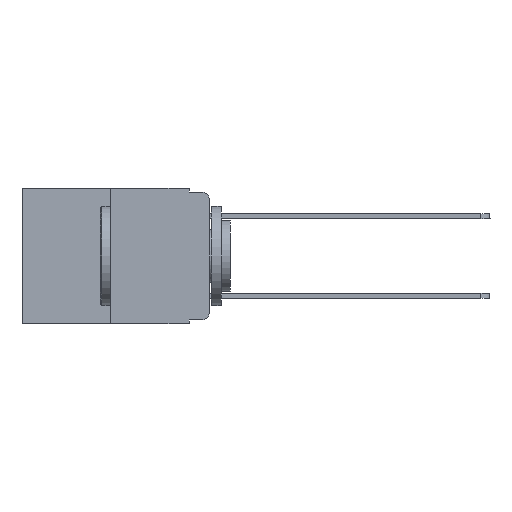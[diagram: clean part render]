
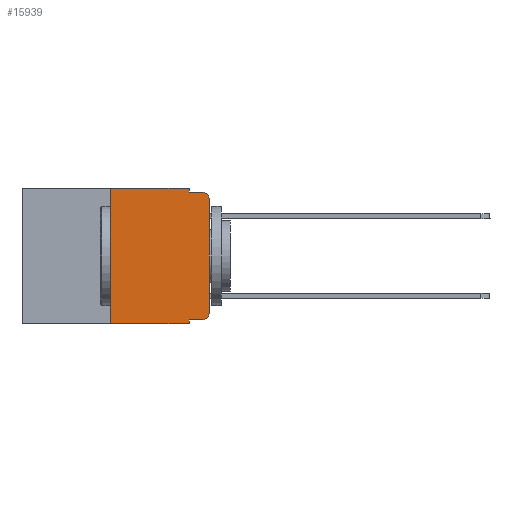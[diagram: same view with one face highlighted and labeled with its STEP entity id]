
A CAD part, left-side view. The second image highlights one B-rep face of the part: STEP entity #15939.
In plain terms, the highlighted planar face has unit normal (-1, 0, 0).
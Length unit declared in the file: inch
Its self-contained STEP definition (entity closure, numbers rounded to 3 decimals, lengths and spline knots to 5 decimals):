
#294 = CARTESIAN_POINT ( 'NONE',  ( 0., 0.02, -0.03 ) ) ;
#412 = CARTESIAN_POINT ( 'NONE',  ( 0., 0.25, 0. ) ) ;
#647 = LINE ( 'NONE', #10317, #19879 ) ;
#972 = VECTOR ( 'NONE', #15878, 39.37008 ) ;
#1545 = EDGE_CURVE ( 'NONE', #7314, #17038, #19181, .T. ) ;
#1686 = VERTEX_POINT ( 'NONE', #6686 ) ;
#2175 = VECTOR ( 'NONE', #7038, 39.37008 ) ;
#2213 = VERTEX_POINT ( 'NONE', #7224 ) ;
#2921 = VECTOR ( 'NONE', #7939, 39.37008 ) ;
#3126 = CIRCLE ( 'NONE', #11602, 0.02 ) ;
#3187 = DIRECTION ( 'NONE',  ( -1., 0., 0. ) ) ;
#3329 = ORIENTED_EDGE ( 'NONE', *, *, #15059, .F. ) ;
#3404 = EDGE_CURVE ( 'NONE', #5990, #1686, #5794, .T. ) ;
#3610 = AXIS2_PLACEMENT_3D ( 'NONE', #5302, #3187, #21129 ) ;
#3692 = CARTESIAN_POINT ( 'NONE',  ( 0., 0.473, -0.343 ) ) ;
#4550 = VECTOR ( 'NONE', #22333, 39.37008 ) ;
#4834 = VERTEX_POINT ( 'NONE', #8156 ) ;
#5104 = VERTEX_POINT ( 'NONE', #17896 ) ;
#5302 = CARTESIAN_POINT ( 'NONE',  ( 0., 0.02, -0.313 ) ) ;
#5708 = ORIENTED_EDGE ( 'NONE', *, *, #1545, .T. ) ;
#5758 = PLANE ( 'NONE',  #7805 ) ;
#5794 = CIRCLE ( 'NONE', #3610, 0.02 ) ;
#5969 = FACE_OUTER_BOUND ( 'NONE', #13307, .T. ) ;
#5990 = VERTEX_POINT ( 'NONE', #6521 ) ;
#6176 = CARTESIAN_POINT ( 'NONE',  ( 0., 0.473, 0. ) ) ;
#6521 = CARTESIAN_POINT ( 'NONE',  ( 0., 0.02, -0.333 ) ) ;
#6523 = CARTESIAN_POINT ( 'NONE',  ( 0., 0.25, -0.343 ) ) ;
#6686 = CARTESIAN_POINT ( 'NONE',  ( 0., 0., -0.313 ) ) ;
#6783 = LINE ( 'NONE', #22415, #4550 ) ;
#6958 = CARTESIAN_POINT ( 'NONE',  ( 0., 0.051, -0.01 ) ) ;
#7038 = DIRECTION ( 'NONE',  ( 0., -1., 0. ) ) ;
#7224 = CARTESIAN_POINT ( 'NONE',  ( 0., 0.051, -0.01 ) ) ;
#7314 = VERTEX_POINT ( 'NONE', #6523 ) ;
#7329 = EDGE_CURVE ( 'NONE', #4834, #5104, #3126, .T. ) ;
#7805 = AXIS2_PLACEMENT_3D ( 'NONE', #9295, #11041, #21880 ) ;
#7939 = DIRECTION ( 'NONE',  ( 0., 0., 1. ) ) ;
#8156 = CARTESIAN_POINT ( 'NONE',  ( 0., 0., -0.03 ) ) ;
#8345 = ORIENTED_EDGE ( 'NONE', *, *, #11212, .F. ) ;
#8813 = LINE ( 'NONE', #9014, #972 ) ;
#9014 = CARTESIAN_POINT ( 'NONE',  ( 0., 0.051, 0. ) ) ;
#9295 = CARTESIAN_POINT ( 'NONE',  ( 0., 0.473, 0. ) ) ;
#9380 = ORIENTED_EDGE ( 'NONE', *, *, #15444, .F. ) ;
#9589 = CARTESIAN_POINT ( 'NONE',  ( 0., 0.051, -0.333 ) ) ;
#10317 = CARTESIAN_POINT ( 'NONE',  ( 0., 0.051, 0. ) ) ;
#11041 = DIRECTION ( 'NONE',  ( 1., 0., 0. ) ) ;
#11212 = EDGE_CURVE ( 'NONE', #15350, #21975, #15100, .T. ) ;
#11302 = ORIENTED_EDGE ( 'NONE', *, *, #12748, .T. ) ;
#11352 = ORIENTED_EDGE ( 'NONE', *, *, #16706, .T. ) ;
#11602 = AXIS2_PLACEMENT_3D ( 'NONE', #294, #21483, #14356 ) ;
#12748 = EDGE_CURVE ( 'NONE', #1686, #4834, #22528, .T. ) ;
#13174 = ORIENTED_EDGE ( 'NONE', *, *, #3404, .T. ) ;
#13307 = EDGE_LOOP ( 'NONE', ( #11302, #13879, #17940, #15015, #8345, #9380, #5708, #3329, #11352, #13174 ) ) ;
#13341 = VECTOR ( 'NONE', #14730, 39.37008 ) ;
#13879 = ORIENTED_EDGE ( 'NONE', *, *, #7329, .T. ) ;
#14356 = DIRECTION ( 'NONE',  ( 0., 0., -1. ) ) ;
#14694 = CARTESIAN_POINT ( 'NONE',  ( 0., 0.25, 0. ) ) ;
#14730 = DIRECTION ( 'NONE',  ( 0., 0., 1. ) ) ;
#15015 = ORIENTED_EDGE ( 'NONE', *, *, #17666, .F. ) ;
#15059 = EDGE_CURVE ( 'NONE', #18977, #17038, #647, .T. ) ;
#15100 = LINE ( 'NONE', #6176, #15673 ) ;
#15132 = EDGE_CURVE ( 'NONE', #2213, #5104, #20431, .T. ) ;
#15350 = VERTEX_POINT ( 'NONE', #14694 ) ;
#15444 = EDGE_CURVE ( 'NONE', #7314, #15350, #16254, .T. ) ;
#15673 = VECTOR ( 'NONE', #20516, 39.37008 ) ;
#15739 = DIRECTION ( 'NONE',  ( 0., 0., -1. ) ) ;
#15809 = CARTESIAN_POINT ( 'NONE',  ( 0., 0.051, 0. ) ) ;
#15878 = DIRECTION ( 'NONE',  ( 0., 0., -1. ) ) ;
#15939 = ADVANCED_FACE ( 'NONE', ( #5969 ), #5758, .F. ) ;
#16025 = VECTOR ( 'NONE', #21160, 39.37008 ) ;
#16254 = LINE ( 'NONE', #412, #2921 ) ;
#16706 = EDGE_CURVE ( 'NONE', #18977, #5990, #6783, .T. ) ;
#17038 = VERTEX_POINT ( 'NONE', #19596 ) ;
#17666 = EDGE_CURVE ( 'NONE', #21975, #2213, #8813, .T. ) ;
#17896 = CARTESIAN_POINT ( 'NONE',  ( 0., 0.02, -0.01 ) ) ;
#17940 = ORIENTED_EDGE ( 'NONE', *, *, #15132, .F. ) ;
#18977 = VERTEX_POINT ( 'NONE', #9589 ) ;
#19181 = LINE ( 'NONE', #3692, #2175 ) ;
#19596 = CARTESIAN_POINT ( 'NONE',  ( 0., 0.051, -0.343 ) ) ;
#19879 = VECTOR ( 'NONE', #15739, 39.37008 ) ;
#20431 = LINE ( 'NONE', #6958, #16025 ) ;
#20516 = DIRECTION ( 'NONE',  ( 0., -1., 0. ) ) ;
#21129 = DIRECTION ( 'NONE',  ( 0., 0., -1. ) ) ;
#21160 = DIRECTION ( 'NONE',  ( 0., -1., 0. ) ) ;
#21483 = DIRECTION ( 'NONE',  ( -1., 0., 0. ) ) ;
#21784 = CARTESIAN_POINT ( 'NONE',  ( 0., 0., 0. ) ) ;
#21880 = DIRECTION ( 'NONE',  ( 0., 0., -1. ) ) ;
#21975 = VERTEX_POINT ( 'NONE', #15809 ) ;
#22333 = DIRECTION ( 'NONE',  ( 0., -1., 0. ) ) ;
#22415 = CARTESIAN_POINT ( 'NONE',  ( 0., 0.051, -0.333 ) ) ;
#22528 = LINE ( 'NONE', #21784, #13341 ) ;
